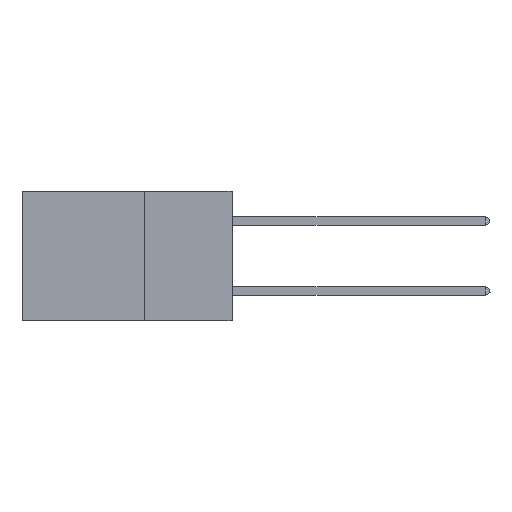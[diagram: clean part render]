
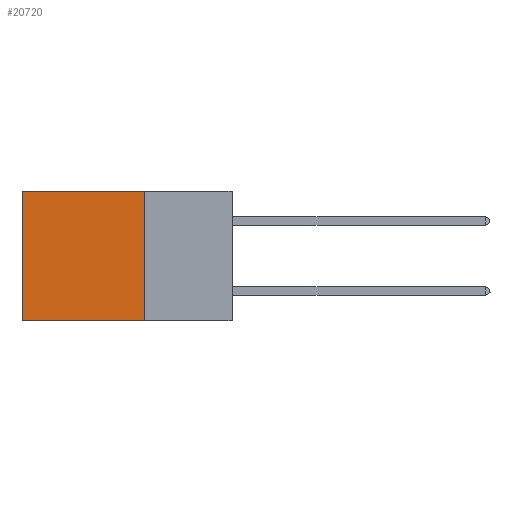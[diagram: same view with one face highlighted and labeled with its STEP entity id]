
A CAD part, left-side view. The second image highlights one B-rep face of the part: STEP entity #20720.
In plain terms, the highlighted planar face has unit normal (-1, 0, 0).
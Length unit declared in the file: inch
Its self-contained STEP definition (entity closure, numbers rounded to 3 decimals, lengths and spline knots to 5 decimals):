
#5 = LINE ( 'NONE', #9580, #24850 ) ;
#477 = VERTEX_POINT ( 'NONE', #19321 ) ;
#1105 = EDGE_LOOP ( 'NONE', ( #3835, #25682, #7733, #2145 ) ) ;
#2058 = CARTESIAN_POINT ( 'NONE',  ( 0.2875, 0.25, -0.37 ) ) ;
#2145 = ORIENTED_EDGE ( 'NONE', *, *, #18040, .T. ) ;
#3835 = ORIENTED_EDGE ( 'NONE', *, *, #6951, .T. ) ;
#4803 = CARTESIAN_POINT ( 'NONE',  ( 0.2875, 0.25, 0. ) ) ;
#5912 = VERTEX_POINT ( 'NONE', #15239 ) ;
#6951 = EDGE_CURVE ( 'NONE', #5912, #477, #12971, .T. ) ;
#7336 = VECTOR ( 'NONE', #15556, 39.37008 ) ;
#7733 = ORIENTED_EDGE ( 'NONE', *, *, #18733, .F. ) ;
#9580 = CARTESIAN_POINT ( 'NONE',  ( 0.2875, 0.25, -0.37 ) ) ;
#10592 = EDGE_CURVE ( 'NONE', #26920, #477, #5, .T. ) ;
#11027 = DIRECTION ( 'NONE',  ( 0., 0., -1. ) ) ;
#11581 = CARTESIAN_POINT ( 'NONE',  ( 0.2875, 0.6, 0. ) ) ;
#11675 = LINE ( 'NONE', #4803, #7336 ) ;
#11733 = DIRECTION ( 'NONE',  ( 0., 1., 0. ) ) ;
#11864 = FACE_OUTER_BOUND ( 'NONE', #1105, .T. ) ;
#12971 = LINE ( 'NONE', #11581, #18625 ) ;
#13717 = DIRECTION ( 'NONE',  ( 0., 0., -1. ) ) ;
#15005 = PLANE ( 'NONE',  #23394 ) ;
#15017 = VECTOR ( 'NONE', #23739, 39.37008 ) ;
#15239 = CARTESIAN_POINT ( 'NONE',  ( 0.2875, 0.6, 0. ) ) ;
#15556 = DIRECTION ( 'NONE',  ( 0., 0., -1. ) ) ;
#17189 = CARTESIAN_POINT ( 'NONE',  ( 0.2875, 0.25, 0. ) ) ;
#18040 = EDGE_CURVE ( 'NONE', #26793, #5912, #22094, .T. ) ;
#18577 = CARTESIAN_POINT ( 'NONE',  ( 0.2875, 0.25, 0. ) ) ;
#18625 = VECTOR ( 'NONE', #13717, 39.37008 ) ;
#18733 = EDGE_CURVE ( 'NONE', #26793, #26920, #11675, .T. ) ;
#19321 = CARTESIAN_POINT ( 'NONE',  ( 0.2875, 0.6, -0.37 ) ) ;
#19361 = DIRECTION ( 'NONE',  ( 1., 0., 0. ) ) ;
#20720 = ADVANCED_FACE ( 'NONE', ( #11864 ), #15005, .F. ) ;
#22094 = LINE ( 'NONE', #25908, #15017 ) ;
#23394 = AXIS2_PLACEMENT_3D ( 'NONE', #17189, #19361, #11027 ) ;
#23739 = DIRECTION ( 'NONE',  ( 0., 1., 0. ) ) ;
#24850 = VECTOR ( 'NONE', #11733, 39.37008 ) ;
#25682 = ORIENTED_EDGE ( 'NONE', *, *, #10592, .F. ) ;
#25908 = CARTESIAN_POINT ( 'NONE',  ( 0.2875, 0.25, 0. ) ) ;
#26793 = VERTEX_POINT ( 'NONE', #18577 ) ;
#26920 = VERTEX_POINT ( 'NONE', #2058 ) ;
